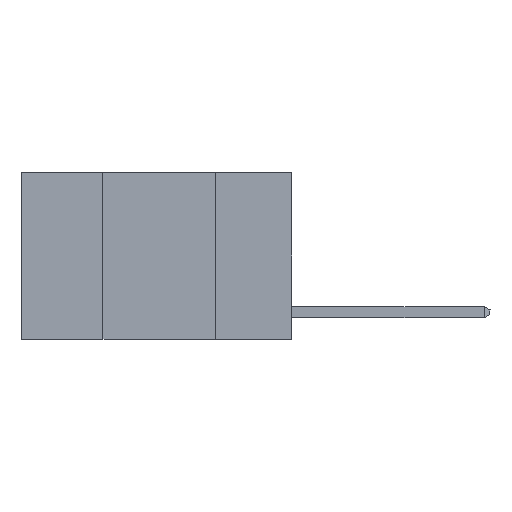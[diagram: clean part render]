
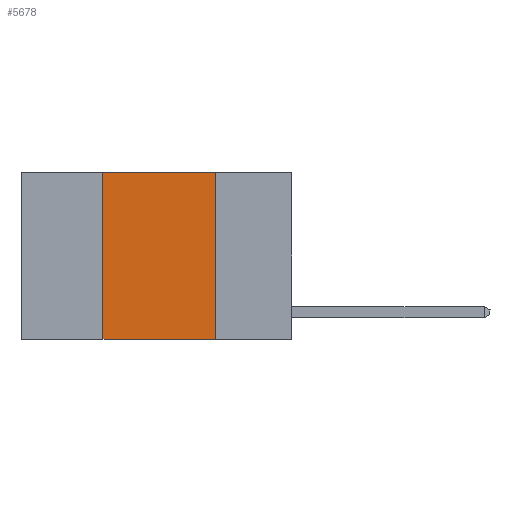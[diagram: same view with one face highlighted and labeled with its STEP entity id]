
A CAD part, left-side view. The second image highlights one B-rep face of the part: STEP entity #5678.
In plain terms, the highlighted planar face has unit normal (-1, 0, 0).
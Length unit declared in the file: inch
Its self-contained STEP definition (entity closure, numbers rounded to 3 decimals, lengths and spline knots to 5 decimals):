
#133 = CARTESIAN_POINT ( 'NONE',  ( 0., 0.17, 0. ) ) ;
#1592 = EDGE_LOOP ( 'NONE', ( #17546, #18128, #22997, #14362 ) ) ;
#2511 = LINE ( 'NONE', #2605, #17691 ) ;
#2605 = CARTESIAN_POINT ( 'NONE',  ( 0., 0.6, -0.37 ) ) ;
#2978 = DIRECTION ( 'NONE',  ( 1., 0., 0. ) ) ;
#3482 = EDGE_CURVE ( 'NONE', #5085, #21322, #2511, .T. ) ;
#3694 = VECTOR ( 'NONE', #6139, 39.37008 ) ;
#3735 = CARTESIAN_POINT ( 'NONE',  ( 0., 0.42, 0. ) ) ;
#4878 = VECTOR ( 'NONE', #11216, 39.37008 ) ;
#5085 = VERTEX_POINT ( 'NONE', #9723 ) ;
#5678 = ADVANCED_FACE ( 'NONE', ( #6318 ), #9399, .F. ) ;
#6139 = DIRECTION ( 'NONE',  ( 0., 0., 1. ) ) ;
#6147 = VERTEX_POINT ( 'NONE', #13181 ) ;
#6318 = FACE_OUTER_BOUND ( 'NONE', #1592, .T. ) ;
#6533 = DIRECTION ( 'NONE',  ( 0., 0., -1. ) ) ;
#7253 = CARTESIAN_POINT ( 'NONE',  ( 0., 0.6, 0. ) ) ;
#9034 = DIRECTION ( 'NONE',  ( 0., -1., 0. ) ) ;
#9164 = EDGE_CURVE ( 'NONE', #6147, #21322, #20497, .T. ) ;
#9274 = CARTESIAN_POINT ( 'NONE',  ( 0., 0.6, 0. ) ) ;
#9330 = LINE ( 'NONE', #23197, #3694 ) ;
#9399 = PLANE ( 'NONE',  #17111 ) ;
#9723 = CARTESIAN_POINT ( 'NONE',  ( 0., 0.42, -0.37 ) ) ;
#11216 = DIRECTION ( 'NONE',  ( 0., -1., 0. ) ) ;
#11323 = DIRECTION ( 'NONE',  ( 0., 0., -1. ) ) ;
#11751 = EDGE_CURVE ( 'NONE', #5085, #23655, #9330, .T. ) ;
#13181 = CARTESIAN_POINT ( 'NONE',  ( 0., 0.17, 0. ) ) ;
#14362 = ORIENTED_EDGE ( 'NONE', *, *, #3482, .T. ) ;
#15984 = LINE ( 'NONE', #9274, #4878 ) ;
#17111 = AXIS2_PLACEMENT_3D ( 'NONE', #7253, #2978, #11323 ) ;
#17546 = ORIENTED_EDGE ( 'NONE', *, *, #9164, .F. ) ;
#17691 = VECTOR ( 'NONE', #9034, 39.37008 ) ;
#17979 = CARTESIAN_POINT ( 'NONE',  ( 0., 0.17, -0.37 ) ) ;
#18128 = ORIENTED_EDGE ( 'NONE', *, *, #19043, .F. ) ;
#19043 = EDGE_CURVE ( 'NONE', #23655, #6147, #15984, .T. ) ;
#20497 = LINE ( 'NONE', #133, #24820 ) ;
#21322 = VERTEX_POINT ( 'NONE', #17979 ) ;
#22997 = ORIENTED_EDGE ( 'NONE', *, *, #11751, .F. ) ;
#23197 = CARTESIAN_POINT ( 'NONE',  ( 0., 0.42, 0. ) ) ;
#23655 = VERTEX_POINT ( 'NONE', #3735 ) ;
#24820 = VECTOR ( 'NONE', #6533, 39.37008 ) ;
